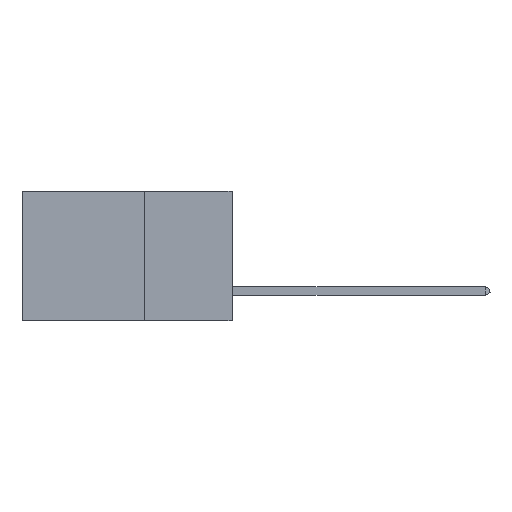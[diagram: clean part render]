
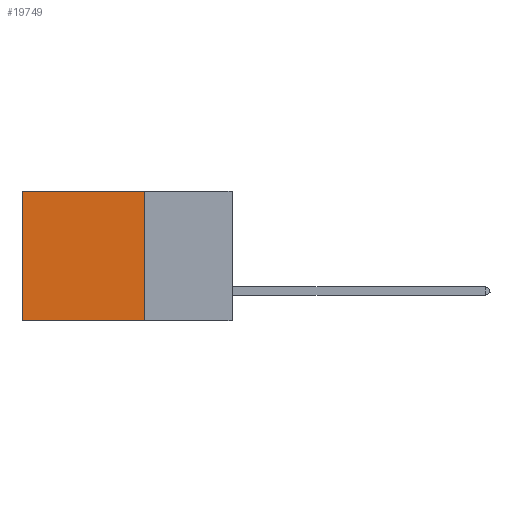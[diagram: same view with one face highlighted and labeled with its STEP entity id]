
A CAD part, left-side view. The second image highlights one B-rep face of the part: STEP entity #19749.
In plain terms, the highlighted planar face has unit normal (-1, 0, 0).
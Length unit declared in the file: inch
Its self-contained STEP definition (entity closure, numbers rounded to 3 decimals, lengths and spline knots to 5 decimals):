
#14 = CARTESIAN_POINT ( 'NONE',  ( 0.2875, 0.6, 0. ) ) ;
#78 = CARTESIAN_POINT ( 'NONE',  ( 0.2875, 0.25, -0.37 ) ) ;
#965 = FACE_OUTER_BOUND ( 'NONE', #11716, .T. ) ;
#1082 = VERTEX_POINT ( 'NONE', #22286 ) ;
#1381 = CARTESIAN_POINT ( 'NONE',  ( 0.2875, 0.25, -0.37 ) ) ;
#2920 = VECTOR ( 'NONE', #9971, 39.37008 ) ;
#3073 = ORIENTED_EDGE ( 'NONE', *, *, #11727, .F. ) ;
#3103 = ORIENTED_EDGE ( 'NONE', *, *, #4670, .T. ) ;
#4244 = DIRECTION ( 'NONE',  ( 0., 0., -1. ) ) ;
#4300 = EDGE_CURVE ( 'NONE', #13595, #1082, #17953, .T. ) ;
#4670 = EDGE_CURVE ( 'NONE', #21680, #1082, #12545, .T. ) ;
#9698 = LINE ( 'NONE', #18722, #2920 ) ;
#9858 = VECTOR ( 'NONE', #13474, 39.37008 ) ;
#9971 = DIRECTION ( 'NONE',  ( 0., 1., 0. ) ) ;
#10243 = CARTESIAN_POINT ( 'NONE',  ( 0.2875, 0.25, 0. ) ) ;
#11460 = AXIS2_PLACEMENT_3D ( 'NONE', #10243, #17128, #18929 ) ;
#11475 = ORIENTED_EDGE ( 'NONE', *, *, #14173, .T. ) ;
#11716 = EDGE_LOOP ( 'NONE', ( #3103, #15479, #3073, #11475 ) ) ;
#11727 = EDGE_CURVE ( 'NONE', #17373, #13595, #22185, .T. ) ;
#12545 = LINE ( 'NONE', #16111, #19031 ) ;
#13474 = DIRECTION ( 'NONE',  ( 0., 1., 0. ) ) ;
#13595 = VERTEX_POINT ( 'NONE', #78 ) ;
#14173 = EDGE_CURVE ( 'NONE', #17373, #21680, #9698, .T. ) ;
#15479 = ORIENTED_EDGE ( 'NONE', *, *, #4300, .F. ) ;
#16111 = CARTESIAN_POINT ( 'NONE',  ( 0.2875, 0.6, 0. ) ) ;
#17128 = DIRECTION ( 'NONE',  ( 1., 0., 0. ) ) ;
#17373 = VERTEX_POINT ( 'NONE', #20351 ) ;
#17881 = VECTOR ( 'NONE', #20967, 39.37008 ) ;
#17953 = LINE ( 'NONE', #1381, #9858 ) ;
#18722 = CARTESIAN_POINT ( 'NONE',  ( 0.2875, 0.25, 0. ) ) ;
#18929 = DIRECTION ( 'NONE',  ( 0., 0., -1. ) ) ;
#19031 = VECTOR ( 'NONE', #4244, 39.37008 ) ;
#19749 = ADVANCED_FACE ( 'NONE', ( #965 ), #20568, .F. ) ;
#20351 = CARTESIAN_POINT ( 'NONE',  ( 0.2875, 0.25, 0. ) ) ;
#20568 = PLANE ( 'NONE',  #11460 ) ;
#20967 = DIRECTION ( 'NONE',  ( 0., 0., -1. ) ) ;
#21680 = VERTEX_POINT ( 'NONE', #14 ) ;
#22096 = CARTESIAN_POINT ( 'NONE',  ( 0.2875, 0.25, 0. ) ) ;
#22185 = LINE ( 'NONE', #22096, #17881 ) ;
#22286 = CARTESIAN_POINT ( 'NONE',  ( 0.2875, 0.6, -0.37 ) ) ;
